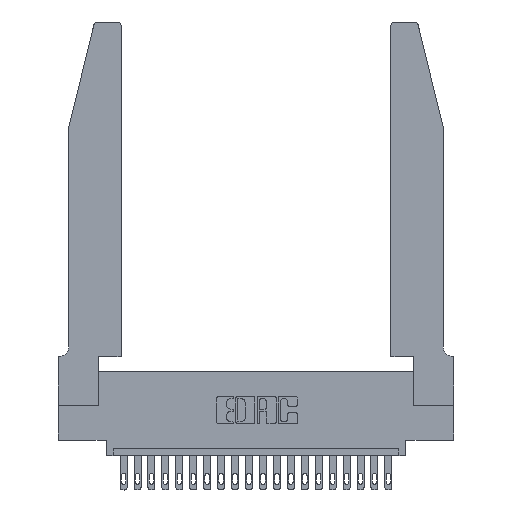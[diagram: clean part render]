
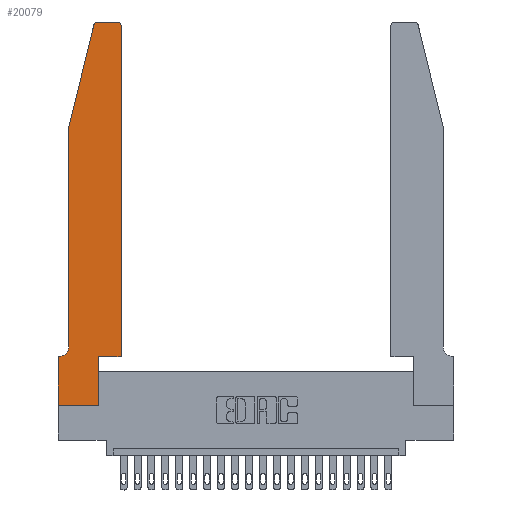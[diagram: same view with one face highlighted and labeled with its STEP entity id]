
A CAD part, top view. The second image highlights one B-rep face of the part: STEP entity #20079.
In plain terms, the highlighted planar face has unit normal (0, 0, 1).
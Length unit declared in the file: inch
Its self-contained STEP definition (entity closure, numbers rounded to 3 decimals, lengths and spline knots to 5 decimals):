
#341 = LINE ( 'NONE', #8816, #10248 ) ;
#472 = FACE_OUTER_BOUND ( 'NONE', #19344, .T. ) ;
#807 = VERTEX_POINT ( 'NONE', #12695 ) ;
#1074 = VECTOR ( 'NONE', #6829, 39.37008 ) ;
#1259 = VECTOR ( 'NONE', #8874, 39.37008 ) ;
#2005 = DIRECTION ( 'NONE',  ( -0.239, -0.971, 0. ) ) ;
#2026 = CARTESIAN_POINT ( 'NONE',  ( 0.2865, 0., 0.37 ) ) ;
#2518 = DIRECTION ( 'NONE',  ( 1., 0., 0. ) ) ;
#2543 = DIRECTION ( 'NONE',  ( 0., 0., -1. ) ) ;
#2721 = LINE ( 'NONE', #5075, #1074 ) ;
#3000 = EDGE_CURVE ( 'NONE', #6436, #4552, #17415, .T. ) ;
#3006 = ORIENTED_EDGE ( 'NONE', *, *, #3000, .T. ) ;
#3141 = EDGE_CURVE ( 'NONE', #3638, #12071, #8910, .T. ) ;
#3368 = CARTESIAN_POINT ( 'NONE',  ( 0., 0.35, 0.37 ) ) ;
#3453 = EDGE_CURVE ( 'NONE', #4552, #17640, #341, .T. ) ;
#3638 = VERTEX_POINT ( 'NONE', #6968 ) ;
#3733 = EDGE_CURVE ( 'NONE', #12071, #11231, #11882, .T. ) ;
#3787 = CARTESIAN_POINT ( 'NONE',  ( 0.284, 2.72, 0.37 ) ) ;
#3794 = CIRCLE ( 'NONE', #21868, 0.03 ) ;
#4308 = DIRECTION ( 'NONE',  ( 0., 0., 1. ) ) ;
#4486 = VERTEX_POINT ( 'NONE', #15575 ) ;
#4552 = VERTEX_POINT ( 'NONE', #20321 ) ;
#4620 = ORIENTED_EDGE ( 'NONE', *, *, #21291, .T. ) ;
#4739 = CARTESIAN_POINT ( 'NONE',  ( 0.2865, 0.35, 0.37 ) ) ;
#4778 = VECTOR ( 'NONE', #10909, 39.37008 ) ;
#4847 = CARTESIAN_POINT ( 'NONE',  ( 0., 0., 0.37 ) ) ;
#5005 = DIRECTION ( 'NONE',  ( 0., 0., 1. ) ) ;
#5070 = LINE ( 'NONE', #16827, #9193 ) ;
#5075 = CARTESIAN_POINT ( 'NONE',  ( 0.2865, 0.35, 0.37 ) ) ;
#5169 = DIRECTION ( 'NONE',  ( 1., 0., 0. ) ) ;
#5211 = CARTESIAN_POINT ( 'NONE',  ( 0., 0., 0.37 ) ) ;
#5306 = EDGE_CURVE ( 'NONE', #12725, #6436, #2721, .T. ) ;
#5489 = ORIENTED_EDGE ( 'NONE', *, *, #5306, .T. ) ;
#5920 = CARTESIAN_POINT ( 'NONE',  ( 0., 0.35, 0.37 ) ) ;
#5977 = LINE ( 'NONE', #14164, #1259 ) ;
#6250 = DIRECTION ( 'NONE',  ( 0., -1., 0. ) ) ;
#6436 = VERTEX_POINT ( 'NONE', #4739 ) ;
#6829 = DIRECTION ( 'NONE',  ( 0., 1., 0. ) ) ;
#6849 = DIRECTION ( 'NONE',  ( -1., 0., 0. ) ) ;
#6968 = CARTESIAN_POINT ( 'NONE',  ( 0.284, 2.75, 0.37 ) ) ;
#7328 = DIRECTION ( 'NONE',  ( 0., 0., 1. ) ) ;
#7361 = LINE ( 'NONE', #15414, #11240 ) ;
#7920 = CARTESIAN_POINT ( 'NONE',  ( 0.4205, 2.72, 0.37 ) ) ;
#8164 = ORIENTED_EDGE ( 'NONE', *, *, #3733, .T. ) ;
#8301 = DIRECTION ( 'NONE',  ( 0., -1., 0. ) ) ;
#8443 = VERTEX_POINT ( 'NONE', #5920 ) ;
#8816 = CARTESIAN_POINT ( 'NONE',  ( 0.4505, 0.35, 0.37 ) ) ;
#8874 = DIRECTION ( 'NONE',  ( -1., 0., 0. ) ) ;
#8879 = ORIENTED_EDGE ( 'NONE', *, *, #12571, .T. ) ;
#8910 = CIRCLE ( 'NONE', #14852, 0.03 ) ;
#8967 = CARTESIAN_POINT ( 'NONE',  ( 0., 0., 0.37 ) ) ;
#9010 = ORIENTED_EDGE ( 'NONE', *, *, #15830, .T. ) ;
#9193 = VECTOR ( 'NONE', #6250, 39.37008 ) ;
#9512 = CARTESIAN_POINT ( 'NONE',  ( 0.4205, 2.75, 0.37 ) ) ;
#10248 = VECTOR ( 'NONE', #14254, 39.37008 ) ;
#10305 = ORIENTED_EDGE ( 'NONE', *, *, #14626, .T. ) ;
#10538 = AXIS2_PLACEMENT_3D ( 'NONE', #3368, #5005, #5169 ) ;
#10908 = CIRCLE ( 'NONE', #22445, 0.07 ) ;
#10909 = DIRECTION ( 'NONE',  ( 1., 0., 0. ) ) ;
#10927 = LINE ( 'NONE', #8967, #16917 ) ;
#11231 = VERTEX_POINT ( 'NONE', #22408 ) ;
#11240 = VECTOR ( 'NONE', #6849, 39.37008 ) ;
#11346 = CARTESIAN_POINT ( 'NONE',  ( 0.0055, 0.42, 0.37 ) ) ;
#11394 = EDGE_CURVE ( 'NONE', #17640, #12889, #3794, .T. ) ;
#11882 = LINE ( 'NONE', #16236, #19881 ) ;
#12071 = VERTEX_POINT ( 'NONE', #17033 ) ;
#12571 = EDGE_CURVE ( 'NONE', #15518, #12725, #10927, .T. ) ;
#12695 = CARTESIAN_POINT ( 'NONE',  ( 0.0755, 0.42, 0.37 ) ) ;
#12725 = VERTEX_POINT ( 'NONE', #2026 ) ;
#12889 = VERTEX_POINT ( 'NONE', #9512 ) ;
#13117 = ORIENTED_EDGE ( 'NONE', *, *, #3141, .T. ) ;
#14164 = CARTESIAN_POINT ( 'NONE',  ( 0.0755, 0.35, 0.37 ) ) ;
#14254 = DIRECTION ( 'NONE',  ( 0., 1., 0. ) ) ;
#14626 = EDGE_CURVE ( 'NONE', #11231, #807, #5070, .T. ) ;
#14829 = ORIENTED_EDGE ( 'NONE', *, *, #20045, .T. ) ;
#14839 = DIRECTION ( 'NONE',  ( -1., 0., 0. ) ) ;
#14852 = AXIS2_PLACEMENT_3D ( 'NONE', #3787, #7328, #2518 ) ;
#15019 = ORIENTED_EDGE ( 'NONE', *, *, #19071, .T. ) ;
#15414 = CARTESIAN_POINT ( 'NONE',  ( 0.2605, 2.75, 0.37 ) ) ;
#15518 = VERTEX_POINT ( 'NONE', #5211 ) ;
#15575 = CARTESIAN_POINT ( 'NONE',  ( 0.0055, 0.35, 0.37 ) ) ;
#15830 = EDGE_CURVE ( 'NONE', #807, #4486, #10908, .T. ) ;
#15916 = LINE ( 'NONE', #4847, #22563 ) ;
#16236 = CARTESIAN_POINT ( 'NONE',  ( 0.0755, 2., 0.37 ) ) ;
#16827 = CARTESIAN_POINT ( 'NONE',  ( 0.0755, 2., 0.37 ) ) ;
#16917 = VECTOR ( 'NONE', #18232, 39.37008 ) ;
#17033 = CARTESIAN_POINT ( 'NONE',  ( 0.25487, 2.72718, 0.37 ) ) ;
#17415 = LINE ( 'NONE', #21685, #4778 ) ;
#17640 = VERTEX_POINT ( 'NONE', #21102 ) ;
#18232 = DIRECTION ( 'NONE',  ( 1., 0., 0. ) ) ;
#18384 = DIRECTION ( 'NONE',  ( 1., 0., 0. ) ) ;
#19071 = EDGE_CURVE ( 'NONE', #8443, #15518, #15916, .T. ) ;
#19344 = EDGE_LOOP ( 'NONE', ( #14829, #13117, #8164, #10305, #9010, #4620, #15019, #8879, #5489, #3006, #21532, #20411 ) ) ;
#19881 = VECTOR ( 'NONE', #2005, 39.37008 ) ;
#20045 = EDGE_CURVE ( 'NONE', #12889, #3638, #7361, .T. ) ;
#20079 = ADVANCED_FACE ( 'NONE', ( #472 ), #20951, .T. ) ;
#20321 = CARTESIAN_POINT ( 'NONE',  ( 0.4505, 0.35, 0.37 ) ) ;
#20411 = ORIENTED_EDGE ( 'NONE', *, *, #11394, .T. ) ;
#20951 = PLANE ( 'NONE',  #10538 ) ;
#21102 = CARTESIAN_POINT ( 'NONE',  ( 0.4505, 2.72, 0.37 ) ) ;
#21291 = EDGE_CURVE ( 'NONE', #4486, #8443, #5977, .T. ) ;
#21532 = ORIENTED_EDGE ( 'NONE', *, *, #3453, .T. ) ;
#21685 = CARTESIAN_POINT ( 'NONE',  ( 0.4505, 0.35, 0.37 ) ) ;
#21868 = AXIS2_PLACEMENT_3D ( 'NONE', #7920, #4308, #18384 ) ;
#22408 = CARTESIAN_POINT ( 'NONE',  ( 0.0755, 2., 0.37 ) ) ;
#22445 = AXIS2_PLACEMENT_3D ( 'NONE', #11346, #2543, #14839 ) ;
#22563 = VECTOR ( 'NONE', #8301, 39.37008 ) ;
